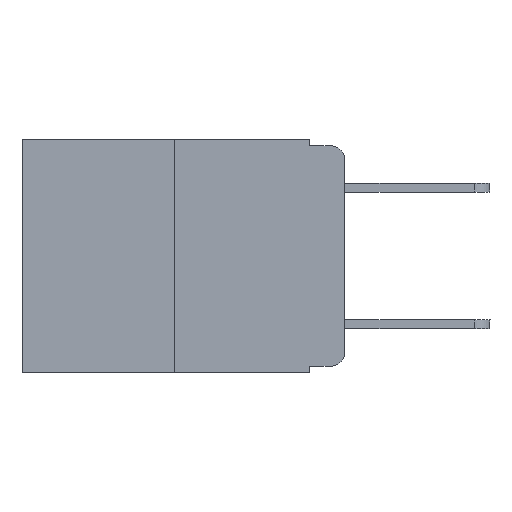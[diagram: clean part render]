
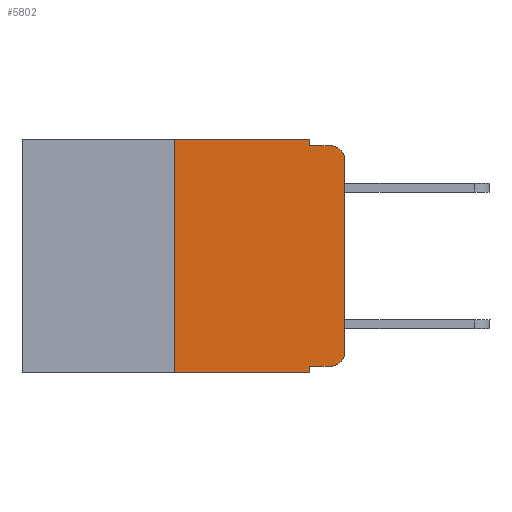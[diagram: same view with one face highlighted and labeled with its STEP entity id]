
A CAD part, left-side view. The second image highlights one B-rep face of the part: STEP entity #5802.
In plain terms, the highlighted planar face has unit normal (-1, 0, 0).
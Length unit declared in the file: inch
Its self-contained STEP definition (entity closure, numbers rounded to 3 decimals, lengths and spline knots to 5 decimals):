
#368 = CARTESIAN_POINT ( 'NONE',  ( 0., 0.051, -0.01 ) ) ;
#549 = VECTOR ( 'NONE', #6987, 39.37008 ) ;
#675 = CARTESIAN_POINT ( 'NONE',  ( 0., 0.051, -0.333 ) ) ;
#728 = CARTESIAN_POINT ( 'NONE',  ( 0., 0.02, -0.01 ) ) ;
#816 = ORIENTED_EDGE ( 'NONE', *, *, #12611, .T. ) ;
#1261 = VERTEX_POINT ( 'NONE', #2300 ) ;
#1390 = LINE ( 'NONE', #5491, #9032 ) ;
#1509 = ORIENTED_EDGE ( 'NONE', *, *, #5925, .F. ) ;
#1883 = CARTESIAN_POINT ( 'NONE',  ( 0., 0.02, -0.313 ) ) ;
#1897 = EDGE_CURVE ( 'NONE', #10909, #13207, #8886, .T. ) ;
#2138 = PLANE ( 'NONE',  #8799 ) ;
#2300 = CARTESIAN_POINT ( 'NONE',  ( 0., 0.25, -0.343 ) ) ;
#2554 = CARTESIAN_POINT ( 'NONE',  ( 0., 0.02, -0.333 ) ) ;
#2627 = DIRECTION ( 'NONE',  ( 0., 0., 1. ) ) ;
#2974 = CARTESIAN_POINT ( 'NONE',  ( 0., 0.25, 0. ) ) ;
#3138 = FACE_OUTER_BOUND ( 'NONE', #5553, .T. ) ;
#3352 = VECTOR ( 'NONE', #11076, 39.37008 ) ;
#3355 = EDGE_CURVE ( 'NONE', #13207, #10700, #1390, .T. ) ;
#3361 = CIRCLE ( 'NONE', #12570, 0.02 ) ;
#3386 = ORIENTED_EDGE ( 'NONE', *, *, #13033, .T. ) ;
#3504 = LINE ( 'NONE', #13210, #549 ) ;
#3593 = ORIENTED_EDGE ( 'NONE', *, *, #4917, .F. ) ;
#3707 = CARTESIAN_POINT ( 'NONE',  ( 0., 0.25, 0. ) ) ;
#3877 = CARTESIAN_POINT ( 'NONE',  ( 0., 0.02, -0.03 ) ) ;
#4008 = LINE ( 'NONE', #6953, #7528 ) ;
#4479 = DIRECTION ( 'NONE',  ( 0., 0., -1. ) ) ;
#4687 = DIRECTION ( 'NONE',  ( 0., -1., 0. ) ) ;
#4745 = CARTESIAN_POINT ( 'NONE',  ( 0., 0.051, -0.343 ) ) ;
#4808 = CIRCLE ( 'NONE', #11636, 0.02 ) ;
#4813 = DIRECTION ( 'NONE',  ( 0., 0., -1. ) ) ;
#4892 = DIRECTION ( 'NONE',  ( 0., 0., -1. ) ) ;
#4907 = DIRECTION ( 'NONE',  ( -1., 0., 0. ) ) ;
#4917 = EDGE_CURVE ( 'NONE', #10700, #8312, #10630, .T. ) ;
#5491 = CARTESIAN_POINT ( 'NONE',  ( 0., 0.051, 0. ) ) ;
#5534 = EDGE_CURVE ( 'NONE', #1261, #10909, #11810, .T. ) ;
#5553 = EDGE_LOOP ( 'NONE', ( #816, #10787, #3593, #12176, #7835, #8565, #10808, #1509, #12767, #3386 ) ) ;
#5792 = VECTOR ( 'NONE', #4687, 39.37008 ) ;
#5802 = ADVANCED_FACE ( 'NONE', ( #3138 ), #2138, .F. ) ;
#5925 = EDGE_CURVE ( 'NONE', #13197, #9988, #4008, .T. ) ;
#6376 = VERTEX_POINT ( 'NONE', #2554 ) ;
#6493 = EDGE_CURVE ( 'NONE', #13197, #6376, #11305, .T. ) ;
#6953 = CARTESIAN_POINT ( 'NONE',  ( 0., 0.051, 0. ) ) ;
#6987 = DIRECTION ( 'NONE',  ( 0., -1., 0. ) ) ;
#7472 = DIRECTION ( 'NONE',  ( 0., -1., 0. ) ) ;
#7494 = CARTESIAN_POINT ( 'NONE',  ( 0., 0.051, 0. ) ) ;
#7528 = VECTOR ( 'NONE', #4813, 39.37008 ) ;
#7686 = DIRECTION ( 'NONE',  ( 1., 0., 0. ) ) ;
#7835 = ORIENTED_EDGE ( 'NONE', *, *, #1897, .F. ) ;
#8009 = DIRECTION ( 'NONE',  ( -1., 0., 0. ) ) ;
#8271 = EDGE_CURVE ( 'NONE', #10712, #8312, #4808, .T. ) ;
#8312 = VERTEX_POINT ( 'NONE', #728 ) ;
#8565 = ORIENTED_EDGE ( 'NONE', *, *, #5534, .F. ) ;
#8799 = AXIS2_PLACEMENT_3D ( 'NONE', #12458, #7686, #12723 ) ;
#8886 = LINE ( 'NONE', #9771, #5792 ) ;
#9018 = CARTESIAN_POINT ( 'NONE',  ( 0., 0., -0.313 ) ) ;
#9032 = VECTOR ( 'NONE', #4479, 39.37008 ) ;
#9259 = CARTESIAN_POINT ( 'NONE',  ( 0., 0., 0. ) ) ;
#9578 = VECTOR ( 'NONE', #7472, 39.37008 ) ;
#9694 = CARTESIAN_POINT ( 'NONE',  ( 0., 0., -0.03 ) ) ;
#9771 = CARTESIAN_POINT ( 'NONE',  ( 0., 0.473, 0. ) ) ;
#9922 = VERTEX_POINT ( 'NONE', #9018 ) ;
#9988 = VERTEX_POINT ( 'NONE', #4745 ) ;
#10080 = VECTOR ( 'NONE', #2627, 39.37008 ) ;
#10454 = CARTESIAN_POINT ( 'NONE',  ( 0., 0.051, -0.333 ) ) ;
#10630 = LINE ( 'NONE', #368, #9578 ) ;
#10700 = VERTEX_POINT ( 'NONE', #10826 ) ;
#10712 = VERTEX_POINT ( 'NONE', #9694 ) ;
#10787 = ORIENTED_EDGE ( 'NONE', *, *, #8271, .T. ) ;
#10808 = ORIENTED_EDGE ( 'NONE', *, *, #11238, .T. ) ;
#10826 = CARTESIAN_POINT ( 'NONE',  ( 0., 0.051, -0.01 ) ) ;
#10909 = VERTEX_POINT ( 'NONE', #2974 ) ;
#11076 = DIRECTION ( 'NONE',  ( 0., 0., 1. ) ) ;
#11238 = EDGE_CURVE ( 'NONE', #1261, #9988, #3504, .T. ) ;
#11305 = LINE ( 'NONE', #675, #12328 ) ;
#11636 = AXIS2_PLACEMENT_3D ( 'NONE', #3877, #8009, #4892 ) ;
#11810 = LINE ( 'NONE', #3707, #10080 ) ;
#12055 = DIRECTION ( 'NONE',  ( 0., -1., 0. ) ) ;
#12144 = LINE ( 'NONE', #9259, #3352 ) ;
#12176 = ORIENTED_EDGE ( 'NONE', *, *, #3355, .F. ) ;
#12328 = VECTOR ( 'NONE', #12055, 39.37008 ) ;
#12458 = CARTESIAN_POINT ( 'NONE',  ( 0., 0.473, 0. ) ) ;
#12570 = AXIS2_PLACEMENT_3D ( 'NONE', #1883, #4907, #13069 ) ;
#12611 = EDGE_CURVE ( 'NONE', #9922, #10712, #12144, .T. ) ;
#12723 = DIRECTION ( 'NONE',  ( 0., 0., -1. ) ) ;
#12767 = ORIENTED_EDGE ( 'NONE', *, *, #6493, .T. ) ;
#13033 = EDGE_CURVE ( 'NONE', #6376, #9922, #3361, .T. ) ;
#13069 = DIRECTION ( 'NONE',  ( 0., 0., -1. ) ) ;
#13197 = VERTEX_POINT ( 'NONE', #10454 ) ;
#13207 = VERTEX_POINT ( 'NONE', #7494 ) ;
#13210 = CARTESIAN_POINT ( 'NONE',  ( 0., 0.473, -0.343 ) ) ;
